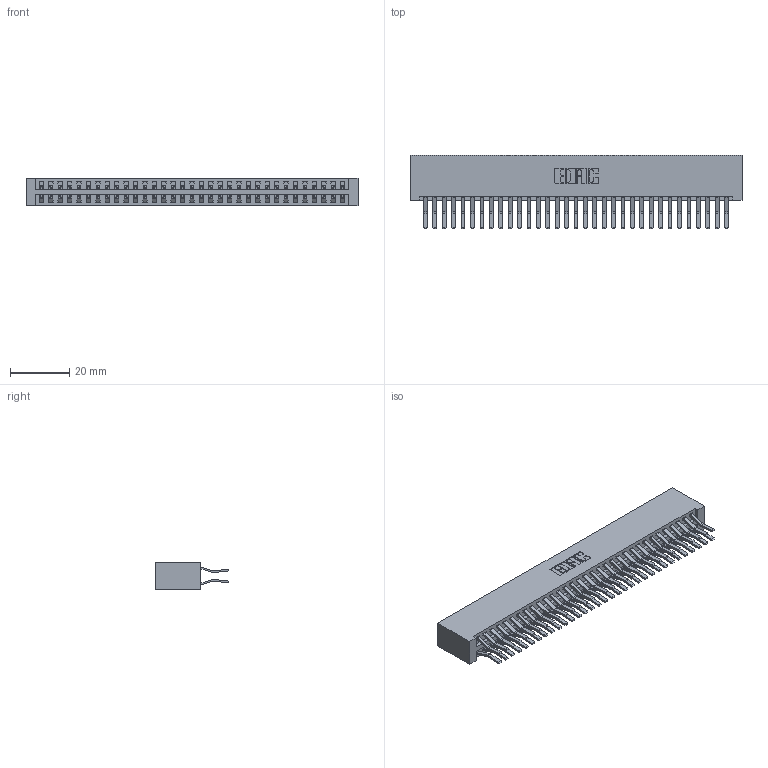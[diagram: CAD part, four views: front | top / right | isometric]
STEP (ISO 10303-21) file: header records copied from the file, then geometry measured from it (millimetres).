
FILE_DESCRIPTION (( 'STEP AP203' ), '1' );
FILE_NAME ('396-066-560-201.STEP', '2018-09-08T20:23:43', ( '' ), ( '' ), 'SwSTEP 2.0', 'SolidWorks 2016', '' );
FILE_SCHEMA (( 'CONFIG_CONTROL_DESIGN' ));
Length unit declared in the file: inch
Products named in the file (3): 345-292-001_560 Tail; 396-066-560-201; 346 Part_No Mounting Lugs
Assembly tree (67 placements, depth 2):
  396-066-560-201
    346 Part_No Mounting Lugs
    345-292-001_560 Tail  x66
Bounding box: 112.01 x 24.78 x 9.4 mm (x, y, z)
Volume: 11858.7 mm3; surface area: 17476.5 mm2
Topology: 67 solids, 67 shells, 3678 faces, 10931 edges, 7198 vertices
Faces by surface type: plane 2382, cylinder 1296
Entity records: 22559 total; most frequent: CARTESIAN_POINT 3728, ORIENTED_EDGE 3662, DIRECTION 3335, EDGE_CURVE 1831, VECTOR 1571, LINE 1571, VERTEX_POINT 1218, AXIS2_PLACEMENT_3D 882
